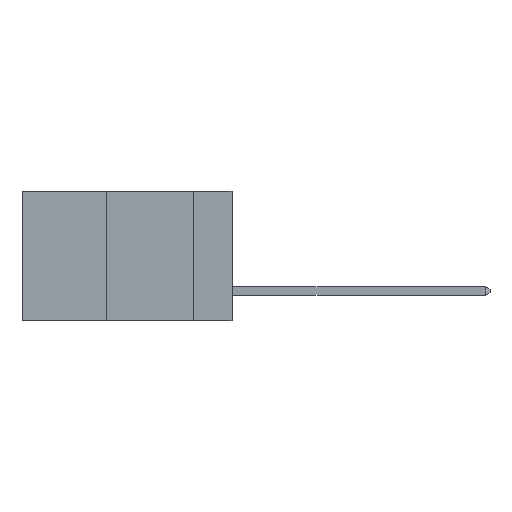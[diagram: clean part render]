
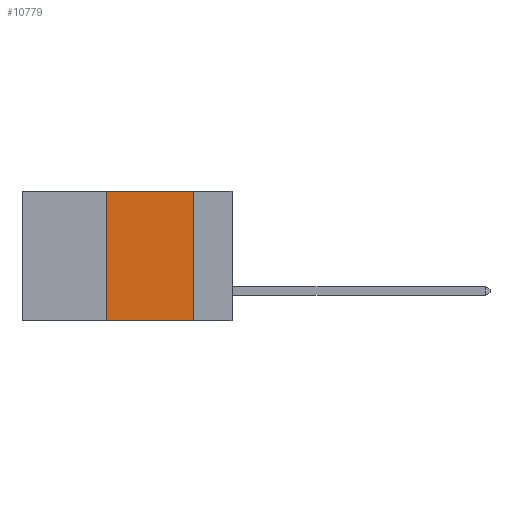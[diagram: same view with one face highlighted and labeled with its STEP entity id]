
A CAD part, left-side view. The second image highlights one B-rep face of the part: STEP entity #10779.
In plain terms, the highlighted planar face has unit normal (-1, 0, 0).
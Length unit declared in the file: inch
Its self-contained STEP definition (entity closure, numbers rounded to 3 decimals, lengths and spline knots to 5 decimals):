
#24 = VERTEX_POINT ( 'NONE', #11384 ) ;
#41 = VECTOR ( 'NONE', #13724, 39.37008 ) ;
#385 = CARTESIAN_POINT ( 'NONE',  ( 0., 0.6, 0. ) ) ;
#1478 = VECTOR ( 'NONE', #13930, 39.37008 ) ;
#1602 = CARTESIAN_POINT ( 'NONE',  ( 0., 0.6, 0. ) ) ;
#1752 = VECTOR ( 'NONE', #13100, 39.37008 ) ;
#2093 = DIRECTION ( 'NONE',  ( 0., 0., -1. ) ) ;
#3376 = EDGE_CURVE ( 'NONE', #3523, #6716, #4611, .T. ) ;
#3523 = VERTEX_POINT ( 'NONE', #11305 ) ;
#4244 = CARTESIAN_POINT ( 'NONE',  ( 0., 0.11, 0. ) ) ;
#4611 = LINE ( 'NONE', #13755, #41 ) ;
#4930 = LINE ( 'NONE', #14569, #9243 ) ;
#4966 = DIRECTION ( 'NONE',  ( 0., 0., 1. ) ) ;
#5781 = LINE ( 'NONE', #1602, #1752 ) ;
#6144 = EDGE_LOOP ( 'NONE', ( #6957, #8371, #8863, #14601 ) ) ;
#6478 = VERTEX_POINT ( 'NONE', #12522 ) ;
#6716 = VERTEX_POINT ( 'NONE', #11568 ) ;
#6957 = ORIENTED_EDGE ( 'NONE', *, *, #8874, .F. ) ;
#6959 = FACE_OUTER_BOUND ( 'NONE', #6144, .T. ) ;
#7801 = EDGE_CURVE ( 'NONE', #3523, #6478, #4930, .T. ) ;
#8371 = ORIENTED_EDGE ( 'NONE', *, *, #14447, .F. ) ;
#8863 = ORIENTED_EDGE ( 'NONE', *, *, #7801, .F. ) ;
#8874 = EDGE_CURVE ( 'NONE', #24, #6716, #14509, .T. ) ;
#9243 = VECTOR ( 'NONE', #4966, 39.37008 ) ;
#10779 = ADVANCED_FACE ( 'NONE', ( #6959 ), #18041, .F. ) ;
#11305 = CARTESIAN_POINT ( 'NONE',  ( 0., 0.36, -0.37 ) ) ;
#11384 = CARTESIAN_POINT ( 'NONE',  ( 0., 0.11, 0. ) ) ;
#11568 = CARTESIAN_POINT ( 'NONE',  ( 0., 0.11, -0.37 ) ) ;
#11959 = DIRECTION ( 'NONE',  ( 1., 0., 0. ) ) ;
#12522 = CARTESIAN_POINT ( 'NONE',  ( 0., 0.36, 0. ) ) ;
#13100 = DIRECTION ( 'NONE',  ( 0., -1., 0. ) ) ;
#13724 = DIRECTION ( 'NONE',  ( 0., -1., 0. ) ) ;
#13755 = CARTESIAN_POINT ( 'NONE',  ( 0., 0.6, -0.37 ) ) ;
#13930 = DIRECTION ( 'NONE',  ( 0., 0., -1. ) ) ;
#14447 = EDGE_CURVE ( 'NONE', #6478, #24, #5781, .T. ) ;
#14509 = LINE ( 'NONE', #4244, #1478 ) ;
#14569 = CARTESIAN_POINT ( 'NONE',  ( 0., 0.36, 0. ) ) ;
#14601 = ORIENTED_EDGE ( 'NONE', *, *, #3376, .T. ) ;
#18041 = PLANE ( 'NONE',  #20208 ) ;
#20208 = AXIS2_PLACEMENT_3D ( 'NONE', #385, #11959, #2093 ) ;
